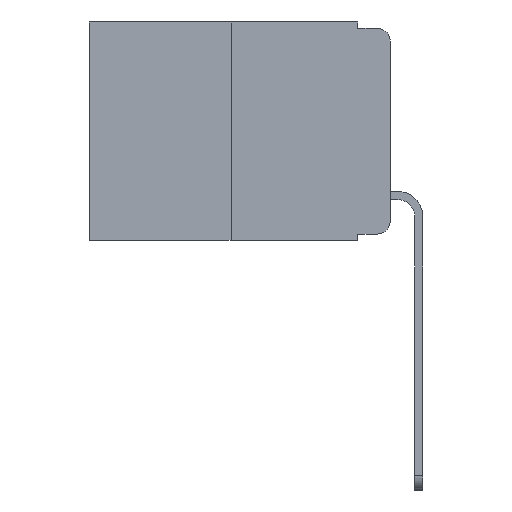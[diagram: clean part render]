
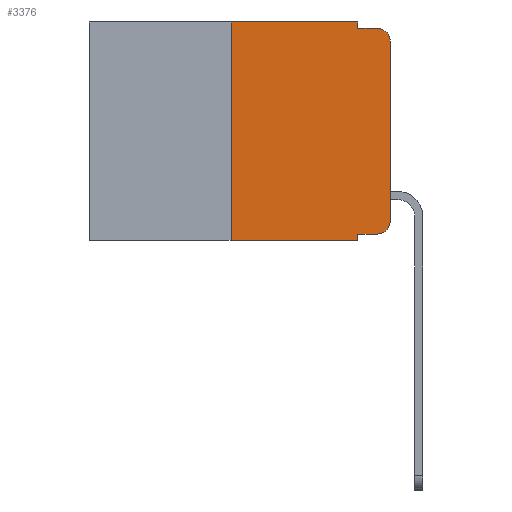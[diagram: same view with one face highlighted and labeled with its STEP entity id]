
A CAD part, left-side view. The second image highlights one B-rep face of the part: STEP entity #3376.
In plain terms, the highlighted planar face has unit normal (-1, 0, 0).
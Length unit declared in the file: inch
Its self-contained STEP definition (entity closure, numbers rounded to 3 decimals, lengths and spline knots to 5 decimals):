
#6 = PLANE ( 'NONE',  #10922 ) ;
#156 = LINE ( 'NONE', #12413, #2640 ) ;
#205 = CARTESIAN_POINT ( 'NONE',  ( 0., 0.051, -0.01 ) ) ;
#322 = CARTESIAN_POINT ( 'NONE',  ( 0., 0., 0. ) ) ;
#387 = CARTESIAN_POINT ( 'NONE',  ( 0., 0.25, 0. ) ) ;
#626 = CARTESIAN_POINT ( 'NONE',  ( 0., 0.25, -0.343 ) ) ;
#689 = VERTEX_POINT ( 'NONE', #15761 ) ;
#1384 = EDGE_CURVE ( 'NONE', #1549, #6976, #7818, .T. ) ;
#1549 = VERTEX_POINT ( 'NONE', #1820 ) ;
#1551 = ORIENTED_EDGE ( 'NONE', *, *, #2254, .T. ) ;
#1651 = DIRECTION ( 'NONE',  ( -1., 0., 0. ) ) ;
#1820 = CARTESIAN_POINT ( 'NONE',  ( 0., 0., -0.03 ) ) ;
#1915 = ORIENTED_EDGE ( 'NONE', *, *, #11282, .F. ) ;
#2165 = AXIS2_PLACEMENT_3D ( 'NONE', #6055, #6230, #14198 ) ;
#2184 = CIRCLE ( 'NONE', #2165, 0.02 ) ;
#2254 = EDGE_CURVE ( 'NONE', #15258, #1549, #12732, .T. ) ;
#2325 = DIRECTION ( 'NONE',  ( 0., 0., -1. ) ) ;
#2640 = VECTOR ( 'NONE', #13814, 39.37008 ) ;
#2657 = DIRECTION ( 'NONE',  ( 0., 0., -1. ) ) ;
#2669 = LINE ( 'NONE', #7150, #7176 ) ;
#2951 = LINE ( 'NONE', #13360, #9111 ) ;
#3046 = LINE ( 'NONE', #16766, #16623 ) ;
#3376 = ADVANCED_FACE ( 'NONE', ( #12894 ), #6, .F. ) ;
#3425 = LINE ( 'NONE', #6542, #3622 ) ;
#3622 = VECTOR ( 'NONE', #10665, 39.37008 ) ;
#3637 = VECTOR ( 'NONE', #9543, 39.37008 ) ;
#3789 = DIRECTION ( 'NONE',  ( 1., 0., 0. ) ) ;
#4678 = VERTEX_POINT ( 'NONE', #7885 ) ;
#5109 = EDGE_CURVE ( 'NONE', #689, #10438, #9924, .T. ) ;
#5599 = DIRECTION ( 'NONE',  ( 0., -1., 0. ) ) ;
#5619 = DIRECTION ( 'NONE',  ( 0., 0., 1. ) ) ;
#5668 = VERTEX_POINT ( 'NONE', #626 ) ;
#6033 = EDGE_CURVE ( 'NONE', #5668, #6160, #2951, .T. ) ;
#6055 = CARTESIAN_POINT ( 'NONE',  ( 0., 0.02, -0.313 ) ) ;
#6149 = CARTESIAN_POINT ( 'NONE',  ( 0., 0.051, -0.01 ) ) ;
#6157 = ORIENTED_EDGE ( 'NONE', *, *, #15443, .F. ) ;
#6160 = VERTEX_POINT ( 'NONE', #387 ) ;
#6230 = DIRECTION ( 'NONE',  ( -1., 0., 0. ) ) ;
#6239 = ORIENTED_EDGE ( 'NONE', *, *, #5109, .T. ) ;
#6542 = CARTESIAN_POINT ( 'NONE',  ( 0., 0.051, 0. ) ) ;
#6976 = VERTEX_POINT ( 'NONE', #9006 ) ;
#7150 = CARTESIAN_POINT ( 'NONE',  ( 0., 0.473, 0. ) ) ;
#7176 = VECTOR ( 'NONE', #9854, 39.37008 ) ;
#7642 = EDGE_LOOP ( 'NONE', ( #1551, #11530, #1915, #12718, #8962, #10708, #13136, #6157, #6239, #8060 ) ) ;
#7818 = CIRCLE ( 'NONE', #14726, 0.02 ) ;
#7885 = CARTESIAN_POINT ( 'NONE',  ( 0., 0.051, 0. ) ) ;
#7930 = CARTESIAN_POINT ( 'NONE',  ( 0., 0.051, -0.343 ) ) ;
#8060 = ORIENTED_EDGE ( 'NONE', *, *, #15801, .T. ) ;
#8294 = VERTEX_POINT ( 'NONE', #7930 ) ;
#8305 = CARTESIAN_POINT ( 'NONE',  ( 0., 0.02, -0.03 ) ) ;
#8723 = EDGE_CURVE ( 'NONE', #4678, #14025, #3046, .T. ) ;
#8962 = ORIENTED_EDGE ( 'NONE', *, *, #11150, .F. ) ;
#9006 = CARTESIAN_POINT ( 'NONE',  ( 0., 0.02, -0.01 ) ) ;
#9111 = VECTOR ( 'NONE', #5619, 39.37008 ) ;
#9543 = DIRECTION ( 'NONE',  ( 0., 0., 1. ) ) ;
#9641 = DIRECTION ( 'NONE',  ( 0., 0., -1. ) ) ;
#9854 = DIRECTION ( 'NONE',  ( 0., -1., 0. ) ) ;
#9924 = LINE ( 'NONE', #12316, #16528 ) ;
#10438 = VERTEX_POINT ( 'NONE', #13633 ) ;
#10578 = DIRECTION ( 'NONE',  ( 0., -1., 0. ) ) ;
#10665 = DIRECTION ( 'NONE',  ( 0., 0., -1. ) ) ;
#10708 = ORIENTED_EDGE ( 'NONE', *, *, #6033, .F. ) ;
#10922 = AXIS2_PLACEMENT_3D ( 'NONE', #11700, #3789, #2657 ) ;
#11150 = EDGE_CURVE ( 'NONE', #6160, #4678, #2669, .T. ) ;
#11282 = EDGE_CURVE ( 'NONE', #14025, #6976, #15502, .T. ) ;
#11530 = ORIENTED_EDGE ( 'NONE', *, *, #1384, .T. ) ;
#11700 = CARTESIAN_POINT ( 'NONE',  ( 0., 0.473, 0. ) ) ;
#12316 = CARTESIAN_POINT ( 'NONE',  ( 0., 0.051, -0.333 ) ) ;
#12413 = CARTESIAN_POINT ( 'NONE',  ( 0., 0.473, -0.343 ) ) ;
#12435 = VECTOR ( 'NONE', #10578, 39.37008 ) ;
#12718 = ORIENTED_EDGE ( 'NONE', *, *, #8723, .F. ) ;
#12732 = LINE ( 'NONE', #322, #3637 ) ;
#12894 = FACE_OUTER_BOUND ( 'NONE', #7642, .T. ) ;
#13136 = ORIENTED_EDGE ( 'NONE', *, *, #15077, .T. ) ;
#13360 = CARTESIAN_POINT ( 'NONE',  ( 0., 0.25, 0. ) ) ;
#13633 = CARTESIAN_POINT ( 'NONE',  ( 0., 0.02, -0.333 ) ) ;
#13814 = DIRECTION ( 'NONE',  ( 0., -1., 0. ) ) ;
#14025 = VERTEX_POINT ( 'NONE', #6149 ) ;
#14198 = DIRECTION ( 'NONE',  ( 0., 0., -1. ) ) ;
#14726 = AXIS2_PLACEMENT_3D ( 'NONE', #8305, #1651, #9641 ) ;
#15077 = EDGE_CURVE ( 'NONE', #5668, #8294, #156, .T. ) ;
#15258 = VERTEX_POINT ( 'NONE', #15587 ) ;
#15443 = EDGE_CURVE ( 'NONE', #689, #8294, #3425, .T. ) ;
#15502 = LINE ( 'NONE', #205, #12435 ) ;
#15587 = CARTESIAN_POINT ( 'NONE',  ( 0., 0., -0.313 ) ) ;
#15761 = CARTESIAN_POINT ( 'NONE',  ( 0., 0.051, -0.333 ) ) ;
#15801 = EDGE_CURVE ( 'NONE', #10438, #15258, #2184, .T. ) ;
#16528 = VECTOR ( 'NONE', #5599, 39.37008 ) ;
#16623 = VECTOR ( 'NONE', #2325, 39.37008 ) ;
#16766 = CARTESIAN_POINT ( 'NONE',  ( 0., 0.051, 0. ) ) ;
